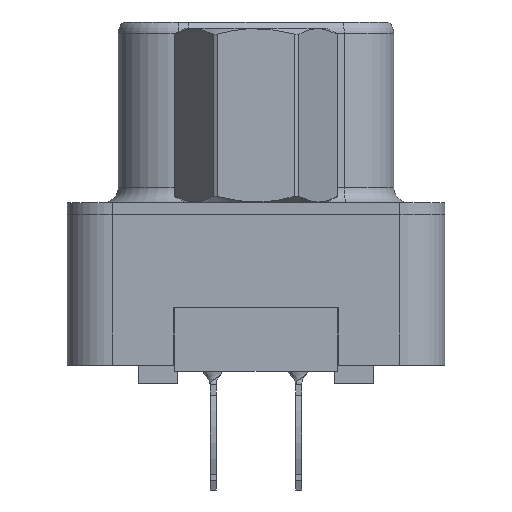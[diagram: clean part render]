
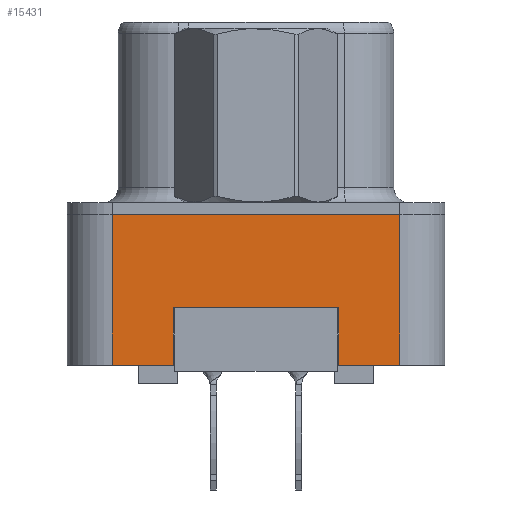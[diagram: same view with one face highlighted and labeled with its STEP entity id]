
A CAD part, left-side view. The second image highlights one B-rep face of the part: STEP entity #15431.
In plain terms, the highlighted planar face has unit normal (-1, 0, 0).
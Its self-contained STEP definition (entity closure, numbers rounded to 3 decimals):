
#678 = VERTEX_POINT ( 'NONE', #20968 ) ;
#801 = DIRECTION ( 'NONE',  ( 0., -1., 0. ) ) ;
#1060 = EDGE_CURVE ( 'NONE', #19709, #15121, #10260, .T. ) ;
#1304 = CARTESIAN_POINT ( 'NONE',  ( -2.91, -4.775, -5. ) ) ;
#1544 = LINE ( 'NONE', #7217, #10333 ) ;
#1760 = EDGE_CURVE ( 'NONE', #18125, #19709, #6558, .T. ) ;
#2596 = CARTESIAN_POINT ( 'NONE',  ( -2.91, -4.775, -5. ) ) ;
#2618 = CARTESIAN_POINT ( 'NONE',  ( -2.91, 2.75, -5. ) ) ;
#2901 = EDGE_CURVE ( 'NONE', #15072, #678, #1544, .T. ) ;
#3067 = CARTESIAN_POINT ( 'NONE',  ( -2.91, 2.75, -3.1 ) ) ;
#3273 = CARTESIAN_POINT ( 'NONE',  ( -2.91, -2.75, -5. ) ) ;
#3318 = CARTESIAN_POINT ( 'NONE',  ( -2.91, -2.75, -3.1 ) ) ;
#3537 = DIRECTION ( 'NONE',  ( 0., 0., -1. ) ) ;
#3931 = CARTESIAN_POINT ( 'NONE',  ( -2.91, -4.775, -5. ) ) ;
#4430 = EDGE_LOOP ( 'NONE', ( #11448, #11665, #14196, #17585, #14537, #14478, #4586, #20031 ) ) ;
#4586 = ORIENTED_EDGE ( 'NONE', *, *, #1060, .F. ) ;
#5064 = VERTEX_POINT ( 'NONE', #12061 ) ;
#5200 = DIRECTION ( 'NONE',  ( 0., 0., 1. ) ) ;
#5936 = VECTOR ( 'NONE', #3537, 1000. ) ;
#6151 = VECTOR ( 'NONE', #801, 1000. ) ;
#6558 = LINE ( 'NONE', #14426, #12530 ) ;
#6567 = EDGE_CURVE ( 'NONE', #18125, #9599, #11531, .T. ) ;
#7217 = CARTESIAN_POINT ( 'NONE',  ( -2.91, -4.775, -5. ) ) ;
#7534 = AXIS2_PLACEMENT_3D ( 'NONE', #2596, #20735, #20948 ) ;
#7789 = DIRECTION ( 'NONE',  ( 0., -1., 0. ) ) ;
#7816 = LINE ( 'NONE', #17741, #6151 ) ;
#8127 = DIRECTION ( 'NONE',  ( 0., 0., 1. ) ) ;
#8474 = CARTESIAN_POINT ( 'NONE',  ( -2.91, -2.75, -3.1 ) ) ;
#9599 = VERTEX_POINT ( 'NONE', #3273 ) ;
#10260 = LINE ( 'NONE', #16826, #10705 ) ;
#10333 = VECTOR ( 'NONE', #8127, 1000. ) ;
#10660 = LINE ( 'NONE', #16907, #12055 ) ;
#10705 = VECTOR ( 'NONE', #13602, 1000. ) ;
#11448 = ORIENTED_EDGE ( 'NONE', *, *, #6567, .T. ) ;
#11531 = LINE ( 'NONE', #3318, #5936 ) ;
#11665 = ORIENTED_EDGE ( 'NONE', *, *, #18331, .T. ) ;
#12055 = VECTOR ( 'NONE', #12282, 1000. ) ;
#12061 = CARTESIAN_POINT ( 'NONE',  ( -2.91, 4.775, 0. ) ) ;
#12282 = DIRECTION ( 'NONE',  ( 0., -1., 0. ) ) ;
#12381 = CARTESIAN_POINT ( 'NONE',  ( -2.91, 4.775, -5. ) ) ;
#12527 = PLANE ( 'NONE',  #7534 ) ;
#12530 = VECTOR ( 'NONE', #21148, 1000. ) ;
#12564 = VERTEX_POINT ( 'NONE', #12381 ) ;
#12576 = EDGE_CURVE ( 'NONE', #12564, #15121, #10660, .T. ) ;
#12666 = VECTOR ( 'NONE', #7789, 1000. ) ;
#13602 = DIRECTION ( 'NONE',  ( 0., 0., -1. ) ) ;
#14142 = FACE_OUTER_BOUND ( 'NONE', #4430, .T. ) ;
#14196 = ORIENTED_EDGE ( 'NONE', *, *, #2901, .T. ) ;
#14426 = CARTESIAN_POINT ( 'NONE',  ( -2.91, 2.75, -3.1 ) ) ;
#14478 = ORIENTED_EDGE ( 'NONE', *, *, #12576, .T. ) ;
#14537 = ORIENTED_EDGE ( 'NONE', *, *, #17708, .F. ) ;
#15072 = VERTEX_POINT ( 'NONE', #3931 ) ;
#15121 = VERTEX_POINT ( 'NONE', #2618 ) ;
#15431 = ADVANCED_FACE ( 'NONE', ( #14142 ), #12527, .T. ) ;
#16826 = CARTESIAN_POINT ( 'NONE',  ( -2.91, 2.75, -3.1 ) ) ;
#16907 = CARTESIAN_POINT ( 'NONE',  ( -2.91, -4.775, -5. ) ) ;
#17585 = ORIENTED_EDGE ( 'NONE', *, *, #18919, .F. ) ;
#17708 = EDGE_CURVE ( 'NONE', #12564, #5064, #19558, .T. ) ;
#17741 = CARTESIAN_POINT ( 'NONE',  ( -2.91, -4.775, 0. ) ) ;
#18125 = VERTEX_POINT ( 'NONE', #8474 ) ;
#18331 = EDGE_CURVE ( 'NONE', #9599, #15072, #20856, .T. ) ;
#18919 = EDGE_CURVE ( 'NONE', #5064, #678, #7816, .T. ) ;
#18920 = VECTOR ( 'NONE', #5200, 1000. ) ;
#19558 = LINE ( 'NONE', #19668, #18920 ) ;
#19668 = CARTESIAN_POINT ( 'NONE',  ( -2.91, 4.775, -5. ) ) ;
#19709 = VERTEX_POINT ( 'NONE', #3067 ) ;
#20031 = ORIENTED_EDGE ( 'NONE', *, *, #1760, .F. ) ;
#20735 = DIRECTION ( 'NONE',  ( -1., 0., 0. ) ) ;
#20856 = LINE ( 'NONE', #1304, #12666 ) ;
#20948 = DIRECTION ( 'NONE',  ( 0., 0., 1. ) ) ;
#20968 = CARTESIAN_POINT ( 'NONE',  ( -2.91, -4.775, 0. ) ) ;
#21148 = DIRECTION ( 'NONE',  ( 0., 1., 0. ) ) ;
